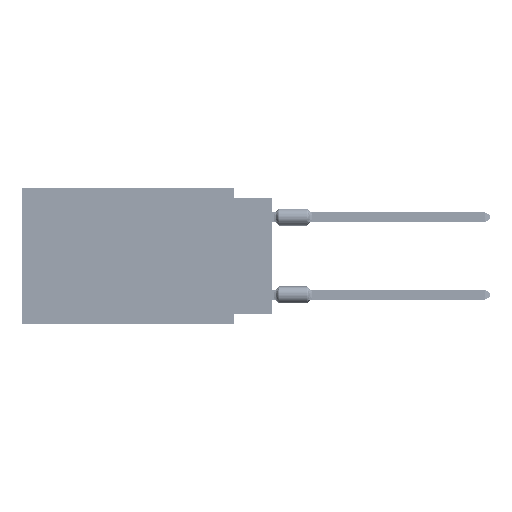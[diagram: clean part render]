
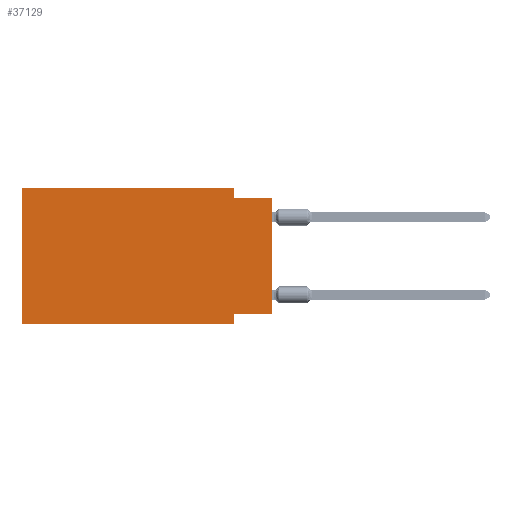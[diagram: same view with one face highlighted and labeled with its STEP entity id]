
A CAD part, left-side view. The second image highlights one B-rep face of the part: STEP entity #37129.
In plain terms, the highlighted planar face has unit normal (-1, 0, 0).
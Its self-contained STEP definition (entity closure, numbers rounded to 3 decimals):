
#1308 = DIRECTION ( 'NONE',  ( 1., 0., 0. ) ) ;
#2732 = VERTEX_POINT ( 'NONE', #29517 ) ;
#3891 = CARTESIAN_POINT ( 'NONE',  ( 0., 0., -0.635 ) ) ;
#5653 = CARTESIAN_POINT ( 'NONE',  ( 0., 2.54, -0.635 ) ) ;
#5858 = LINE ( 'NONE', #74108, #44411 ) ;
#7410 = PLANE ( 'NONE',  #61452 ) ;
#8533 = VECTOR ( 'NONE', #46055, 1000. ) ;
#9119 = LINE ( 'NONE', #32370, #74989 ) ;
#9487 = EDGE_LOOP ( 'NONE', ( #19706, #27567, #25824, #63353, #58059, #49528, #11317, #43516 ) ) ;
#11173 = CARTESIAN_POINT ( 'NONE',  ( 0., 0., 0. ) ) ;
#11317 = ORIENTED_EDGE ( 'NONE', *, *, #49070, .F. ) ;
#14067 = EDGE_CURVE ( 'NONE', #2732, #38705, #47748, .T. ) ;
#15238 = LINE ( 'NONE', #38492, #53920 ) ;
#17649 = CARTESIAN_POINT ( 'NONE',  ( 0., 16.383, 0. ) ) ;
#17673 = DIRECTION ( 'NONE',  ( 0., -1., 0. ) ) ;
#18688 = VECTOR ( 'NONE', #35551, 1000. ) ;
#19221 = CARTESIAN_POINT ( 'NONE',  ( 0., 16.383, 0. ) ) ;
#19706 = ORIENTED_EDGE ( 'NONE', *, *, #70843, .T. ) ;
#21647 = CARTESIAN_POINT ( 'NONE',  ( 0., 2.54, -8.255 ) ) ;
#25321 = DIRECTION ( 'NONE',  ( 0., 0., -1. ) ) ;
#25824 = ORIENTED_EDGE ( 'NONE', *, *, #67860, .F. ) ;
#27393 = VECTOR ( 'NONE', #61789, 1000. ) ;
#27567 = ORIENTED_EDGE ( 'NONE', *, *, #40262, .F. ) ;
#28315 = CARTESIAN_POINT ( 'NONE',  ( 0., 2.54, 0. ) ) ;
#28902 = CARTESIAN_POINT ( 'NONE',  ( 0., 0., -8.255 ) ) ;
#29517 = CARTESIAN_POINT ( 'NONE',  ( 0., 16.383, 0. ) ) ;
#29554 = VECTOR ( 'NONE', #40299, 1000. ) ;
#30202 = EDGE_CURVE ( 'NONE', #44167, #2732, #33509, .T. ) ;
#32370 = CARTESIAN_POINT ( 'NONE',  ( 0., 0., -0.635 ) ) ;
#33509 = LINE ( 'NONE', #39978, #29554 ) ;
#34295 = EDGE_CURVE ( 'NONE', #44167, #42710, #5858, .T. ) ;
#35551 = DIRECTION ( 'NONE',  ( 0., 0., 1. ) ) ;
#37129 = ADVANCED_FACE ( 'NONE', ( #53907 ), #7410, .F. ) ;
#37851 = CARTESIAN_POINT ( 'NONE',  ( 0., 2.54, -8.89 ) ) ;
#38492 = CARTESIAN_POINT ( 'NONE',  ( 0., 2.54, 0. ) ) ;
#38705 = VERTEX_POINT ( 'NONE', #28315 ) ;
#39978 = CARTESIAN_POINT ( 'NONE',  ( 0., 16.383, 0. ) ) ;
#40262 = EDGE_CURVE ( 'NONE', #49216, #63804, #9119, .T. ) ;
#40299 = DIRECTION ( 'NONE',  ( 0., 0., 1. ) ) ;
#40900 = LINE ( 'NONE', #11173, #18688 ) ;
#42274 = CARTESIAN_POINT ( 'NONE',  ( 0., 16.383, -8.89 ) ) ;
#42710 = VERTEX_POINT ( 'NONE', #37851 ) ;
#43516 = ORIENTED_EDGE ( 'NONE', *, *, #59036, .F. ) ;
#44167 = VERTEX_POINT ( 'NONE', #42274 ) ;
#44261 = CARTESIAN_POINT ( 'NONE',  ( 0., 0., -8.255 ) ) ;
#44411 = VECTOR ( 'NONE', #17673, 1000. ) ;
#46055 = DIRECTION ( 'NONE',  ( 0., 0., -1. ) ) ;
#47748 = LINE ( 'NONE', #17649, #64046 ) ;
#49070 = EDGE_CURVE ( 'NONE', #55129, #42710, #62454, .T. ) ;
#49216 = VERTEX_POINT ( 'NONE', #5653 ) ;
#49225 = VERTEX_POINT ( 'NONE', #28902 ) ;
#49528 = ORIENTED_EDGE ( 'NONE', *, *, #34295, .T. ) ;
#50748 = LINE ( 'NONE', #44261, #27393 ) ;
#53907 = FACE_OUTER_BOUND ( 'NONE', #9487, .T. ) ;
#53920 = VECTOR ( 'NONE', #63218, 1000. ) ;
#55129 = VERTEX_POINT ( 'NONE', #21647 ) ;
#57126 = CARTESIAN_POINT ( 'NONE',  ( 0., 2.54, -8.89 ) ) ;
#58059 = ORIENTED_EDGE ( 'NONE', *, *, #30202, .F. ) ;
#58791 = DIRECTION ( 'NONE',  ( 0., -1., 0. ) ) ;
#59036 = EDGE_CURVE ( 'NONE', #49225, #55129, #50748, .T. ) ;
#61452 = AXIS2_PLACEMENT_3D ( 'NONE', #19221, #1308, #25321 ) ;
#61716 = DIRECTION ( 'NONE',  ( 0., -1., 0. ) ) ;
#61789 = DIRECTION ( 'NONE',  ( 0., 1., 0. ) ) ;
#62454 = LINE ( 'NONE', #57126, #8533 ) ;
#63218 = DIRECTION ( 'NONE',  ( 0., 0., -1. ) ) ;
#63353 = ORIENTED_EDGE ( 'NONE', *, *, #14067, .F. ) ;
#63804 = VERTEX_POINT ( 'NONE', #3891 ) ;
#64046 = VECTOR ( 'NONE', #58791, 1000. ) ;
#67860 = EDGE_CURVE ( 'NONE', #38705, #49216, #15238, .T. ) ;
#70843 = EDGE_CURVE ( 'NONE', #49225, #63804, #40900, .T. ) ;
#74108 = CARTESIAN_POINT ( 'NONE',  ( 0., 16.383, -8.89 ) ) ;
#74989 = VECTOR ( 'NONE', #61716, 1000. ) ;
